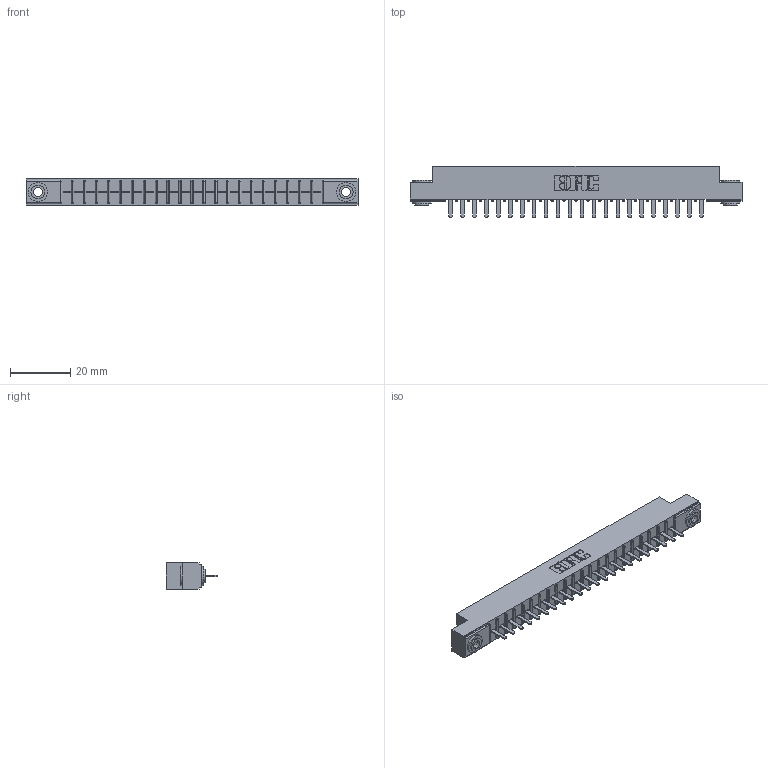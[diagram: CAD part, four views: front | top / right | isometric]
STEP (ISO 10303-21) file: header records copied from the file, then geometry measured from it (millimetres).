
FILE_DESCRIPTION (( 'STEP AP203' ), '1' );
FILE_NAME ('306-022-520-103.STEP', '2019-09-11T20:59:08', ( '' ), ( '' ), 'SwSTEP 2.0', 'SolidWorks 2016', '' );
FILE_SCHEMA (( 'CONFIG_CONTROL_DESIGN' ));
Length unit declared in the file: inch
Products named in the file (4): 306-022-520-103; 345-250-002_345-250-002-102; 306 Part_.156 Dia; 306-290-001_120
Assembly tree (25 placements, depth 2):
  306-022-520-103
    306 Part_.156 Dia
    306-290-001_120  x22
    345-250-002_345-250-002-102  x2
Bounding box: 110.19 x 17.12 x 8.71 mm (x, y, z)
Volume: 7536.3 mm3; surface area: 11406.9 mm2
Topology: 25 solids, 25 shells, 1708 faces, 4762 edges, 3052 vertices
Faces by surface type: plane 1126, cylinder 486, sphere 88, cone 8
Entity records: 24128 total; most frequent: CARTESIAN_POINT 4026, DIRECTION 3986, ORIENTED_EDGE 3980, EDGE_CURVE 1990, VECTOR 1538, LINE 1538, VERTEX_POINT 1264, AXIS2_PLACEMENT_3D 1224
